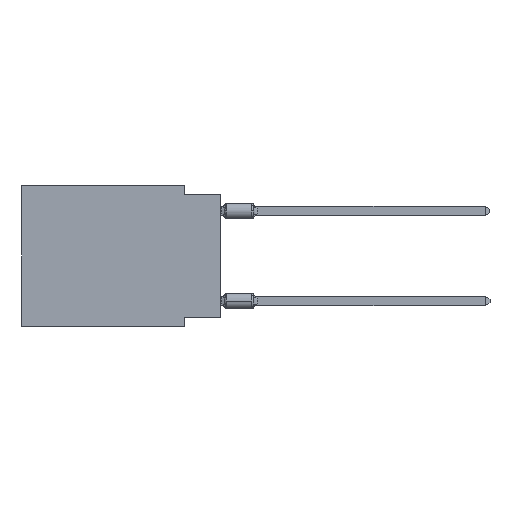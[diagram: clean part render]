
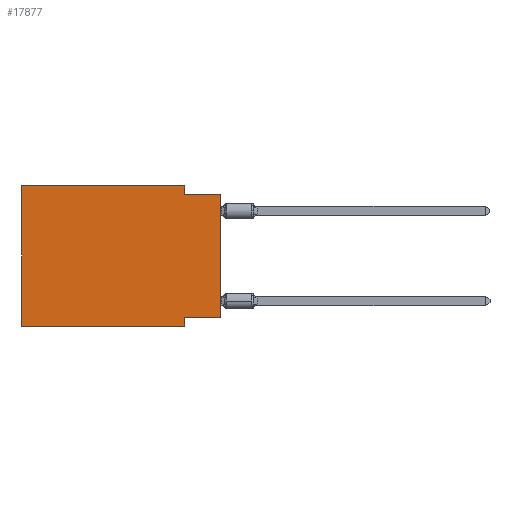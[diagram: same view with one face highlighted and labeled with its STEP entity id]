
A CAD part, left-side view. The second image highlights one B-rep face of the part: STEP entity #17877.
In plain terms, the highlighted planar face has unit normal (-1, 0, 0).
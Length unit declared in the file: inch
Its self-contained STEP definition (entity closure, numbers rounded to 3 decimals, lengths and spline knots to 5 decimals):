
#90 = ORIENTED_EDGE ( 'NONE', *, *, #19532, .T. ) ;
#435 = PLANE ( 'NONE',  #2015 ) ;
#501 = ORIENTED_EDGE ( 'NONE', *, *, #16849, .F. ) ;
#1142 = DIRECTION ( 'NONE',  ( 0., -1., 0. ) ) ;
#1209 = CARTESIAN_POINT ( 'NONE',  ( 0., 0., -0.025 ) ) ;
#2015 = AXIS2_PLACEMENT_3D ( 'NONE', #11057, #28192, #13855 ) ;
#3679 = VECTOR ( 'NONE', #33384, 39.37008 ) ;
#3849 = ORIENTED_EDGE ( 'NONE', *, *, #35351, .F. ) ;
#4856 = EDGE_CURVE ( 'NONE', #13690, #28115, #34751, .T. ) ;
#5576 = EDGE_CURVE ( 'NONE', #6727, #29968, #13848, .T. ) ;
#6135 = DIRECTION ( 'NONE',  ( 0., 0., -1. ) ) ;
#6206 = LINE ( 'NONE', #11970, #10349 ) ;
#6695 = EDGE_CURVE ( 'NONE', #13690, #30328, #9503, .T. ) ;
#6712 = CARTESIAN_POINT ( 'NONE',  ( 0., 0., 0. ) ) ;
#6727 = VERTEX_POINT ( 'NONE', #29624 ) ;
#7930 = VERTEX_POINT ( 'NONE', #9694 ) ;
#8158 = ORIENTED_EDGE ( 'NONE', *, *, #35189, .F. ) ;
#8928 = LINE ( 'NONE', #34595, #20389 ) ;
#9503 = LINE ( 'NONE', #6712, #11593 ) ;
#9694 = CARTESIAN_POINT ( 'NONE',  ( 0., 0.1, -0.39 ) ) ;
#10349 = VECTOR ( 'NONE', #22988, 39.37008 ) ;
#11057 = CARTESIAN_POINT ( 'NONE',  ( 0., 0.55, 0. ) ) ;
#11593 = VECTOR ( 'NONE', #18420, 39.37008 ) ;
#11970 = CARTESIAN_POINT ( 'NONE',  ( 0., 0.1, -0.39 ) ) ;
#12233 = CARTESIAN_POINT ( 'NONE',  ( 0., 0., -0.365 ) ) ;
#12785 = CARTESIAN_POINT ( 'NONE',  ( 0., 0.55, 0. ) ) ;
#13690 = VERTEX_POINT ( 'NONE', #19348 ) ;
#13848 = LINE ( 'NONE', #25221, #3679 ) ;
#13855 = DIRECTION ( 'NONE',  ( 0., 0., -1. ) ) ;
#13970 = CARTESIAN_POINT ( 'NONE',  ( 0., 0.55, 0. ) ) ;
#16849 = EDGE_CURVE ( 'NONE', #35079, #27802, #8928, .T. ) ;
#17771 = CARTESIAN_POINT ( 'NONE',  ( 0., 0.1, -0.365 ) ) ;
#17877 = ADVANCED_FACE ( 'NONE', ( #20174 ), #435, .F. ) ;
#17905 = CARTESIAN_POINT ( 'NONE',  ( 0., 0.1, 0. ) ) ;
#18420 = DIRECTION ( 'NONE',  ( 0., 0., 1. ) ) ;
#19348 = CARTESIAN_POINT ( 'NONE',  ( 0., 0., -0.365 ) ) ;
#19532 = EDGE_CURVE ( 'NONE', #6727, #7930, #19953, .T. ) ;
#19953 = LINE ( 'NONE', #25909, #30078 ) ;
#20174 = FACE_OUTER_BOUND ( 'NONE', #35834, .T. ) ;
#20389 = VECTOR ( 'NONE', #6135, 39.37008 ) ;
#21228 = VECTOR ( 'NONE', #23289, 39.37008 ) ;
#21814 = VECTOR ( 'NONE', #1142, 39.37008 ) ;
#22914 = LINE ( 'NONE', #13970, #21228 ) ;
#22988 = DIRECTION ( 'NONE',  ( 0., 0., -1. ) ) ;
#23289 = DIRECTION ( 'NONE',  ( 0., -1., 0. ) ) ;
#23700 = CARTESIAN_POINT ( 'NONE',  ( 0., 0., -0.025 ) ) ;
#25221 = CARTESIAN_POINT ( 'NONE',  ( 0., 0.55, 0. ) ) ;
#25909 = CARTESIAN_POINT ( 'NONE',  ( 0., 0.55, -0.39 ) ) ;
#27035 = LINE ( 'NONE', #23700, #21814 ) ;
#27802 = VERTEX_POINT ( 'NONE', #35107 ) ;
#28115 = VERTEX_POINT ( 'NONE', #17771 ) ;
#28192 = DIRECTION ( 'NONE',  ( 1., 0., 0. ) ) ;
#28462 = DIRECTION ( 'NONE',  ( 0., 1., 0. ) ) ;
#29049 = ORIENTED_EDGE ( 'NONE', *, *, #30608, .F. ) ;
#29624 = CARTESIAN_POINT ( 'NONE',  ( 0., 0.55, -0.39 ) ) ;
#29883 = ORIENTED_EDGE ( 'NONE', *, *, #4856, .F. ) ;
#29968 = VERTEX_POINT ( 'NONE', #12785 ) ;
#30078 = VECTOR ( 'NONE', #31317, 39.37008 ) ;
#30328 = VERTEX_POINT ( 'NONE', #1209 ) ;
#30439 = VECTOR ( 'NONE', #28462, 39.37008 ) ;
#30608 = EDGE_CURVE ( 'NONE', #28115, #7930, #6206, .T. ) ;
#31317 = DIRECTION ( 'NONE',  ( 0., -1., 0. ) ) ;
#33384 = DIRECTION ( 'NONE',  ( 0., 0., 1. ) ) ;
#34026 = ORIENTED_EDGE ( 'NONE', *, *, #5576, .F. ) ;
#34516 = ORIENTED_EDGE ( 'NONE', *, *, #6695, .T. ) ;
#34595 = CARTESIAN_POINT ( 'NONE',  ( 0., 0.1, 0. ) ) ;
#34751 = LINE ( 'NONE', #12233, #30439 ) ;
#35079 = VERTEX_POINT ( 'NONE', #17905 ) ;
#35107 = CARTESIAN_POINT ( 'NONE',  ( 0., 0.1, -0.025 ) ) ;
#35189 = EDGE_CURVE ( 'NONE', #27802, #30328, #27035, .T. ) ;
#35351 = EDGE_CURVE ( 'NONE', #29968, #35079, #22914, .T. ) ;
#35834 = EDGE_LOOP ( 'NONE', ( #34516, #8158, #501, #3849, #34026, #90, #29049, #29883 ) ) ;
